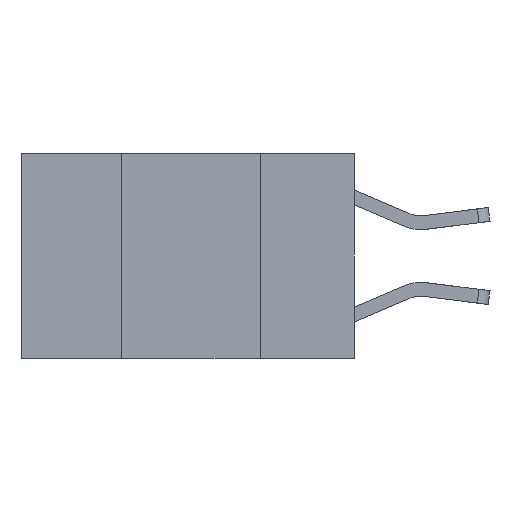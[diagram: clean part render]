
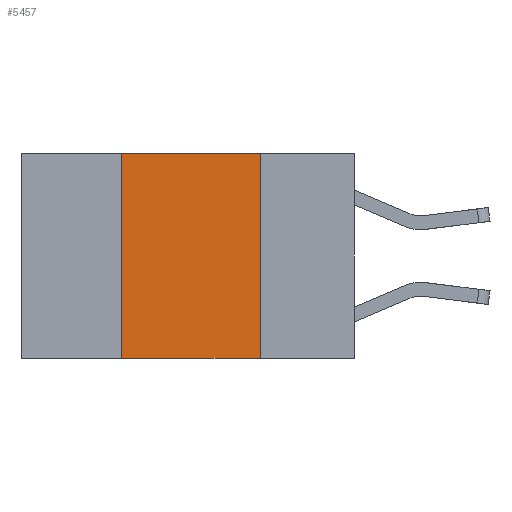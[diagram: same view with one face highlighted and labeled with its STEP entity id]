
A CAD part, left-side view. The second image highlights one B-rep face of the part: STEP entity #5457.
In plain terms, the highlighted planar face has unit normal (-1, 0, 0).
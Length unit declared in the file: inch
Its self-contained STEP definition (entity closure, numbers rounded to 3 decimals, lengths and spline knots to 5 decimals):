
#213 = ORIENTED_EDGE ( 'NONE', *, *, #7279, .F. ) ;
#554 = CARTESIAN_POINT ( 'NONE',  ( 0., 0.42, 0. ) ) ;
#1180 = DIRECTION ( 'NONE',  ( 0., 0., -1. ) ) ;
#1487 = EDGE_CURVE ( 'NONE', #5625, #1554, #8868, .T. ) ;
#1554 = VERTEX_POINT ( 'NONE', #10926 ) ;
#1644 = LINE ( 'NONE', #7925, #8400 ) ;
#1703 = DIRECTION ( 'NONE',  ( 0., 0., -1. ) ) ;
#3079 = EDGE_CURVE ( 'NONE', #1554, #11957, #5678, .T. ) ;
#3225 = PLANE ( 'NONE',  #8171 ) ;
#3305 = EDGE_CURVE ( 'NONE', #5625, #11986, #4185, .T. ) ;
#3471 = VECTOR ( 'NONE', #4811, 39.37008 ) ;
#4161 = VECTOR ( 'NONE', #4247, 39.37008 ) ;
#4185 = LINE ( 'NONE', #7876, #3471 ) ;
#4188 = FACE_OUTER_BOUND ( 'NONE', #8067, .T. ) ;
#4247 = DIRECTION ( 'NONE',  ( 0., 0., 1. ) ) ;
#4811 = DIRECTION ( 'NONE',  ( 0., -1., 0. ) ) ;
#4983 = DIRECTION ( 'NONE',  ( 1., 0., 0. ) ) ;
#5457 = ADVANCED_FACE ( 'NONE', ( #4188 ), #3225, .F. ) ;
#5615 = DIRECTION ( 'NONE',  ( 0., -1., 0. ) ) ;
#5625 = VERTEX_POINT ( 'NONE', #10796 ) ;
#5678 = LINE ( 'NONE', #8392, #6710 ) ;
#5790 = ORIENTED_EDGE ( 'NONE', *, *, #3305, .T. ) ;
#5807 = ORIENTED_EDGE ( 'NONE', *, *, #1487, .F. ) ;
#6019 = CARTESIAN_POINT ( 'NONE',  ( 0., 0.6, 0. ) ) ;
#6430 = CARTESIAN_POINT ( 'NONE',  ( 0., 0.17, -0.37 ) ) ;
#6710 = VECTOR ( 'NONE', #5615, 39.37008 ) ;
#7273 = CARTESIAN_POINT ( 'NONE',  ( 0., 0.17, 0. ) ) ;
#7279 = EDGE_CURVE ( 'NONE', #11957, #11986, #1644, .T. ) ;
#7876 = CARTESIAN_POINT ( 'NONE',  ( 0., 0.6, -0.37 ) ) ;
#7925 = CARTESIAN_POINT ( 'NONE',  ( 0., 0.17, 0. ) ) ;
#8067 = EDGE_LOOP ( 'NONE', ( #213, #11974, #5807, #5790 ) ) ;
#8171 = AXIS2_PLACEMENT_3D ( 'NONE', #6019, #4983, #1180 ) ;
#8392 = CARTESIAN_POINT ( 'NONE',  ( 0., 0.6, 0. ) ) ;
#8400 = VECTOR ( 'NONE', #1703, 39.37008 ) ;
#8868 = LINE ( 'NONE', #554, #4161 ) ;
#10796 = CARTESIAN_POINT ( 'NONE',  ( 0., 0.42, -0.37 ) ) ;
#10926 = CARTESIAN_POINT ( 'NONE',  ( 0., 0.42, 0. ) ) ;
#11957 = VERTEX_POINT ( 'NONE', #7273 ) ;
#11974 = ORIENTED_EDGE ( 'NONE', *, *, #3079, .F. ) ;
#11986 = VERTEX_POINT ( 'NONE', #6430 ) ;
